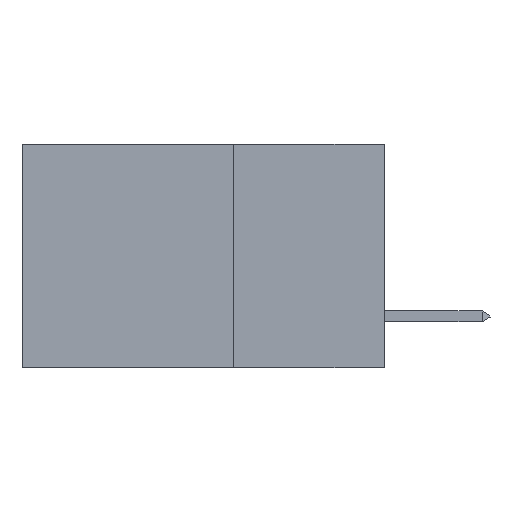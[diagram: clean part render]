
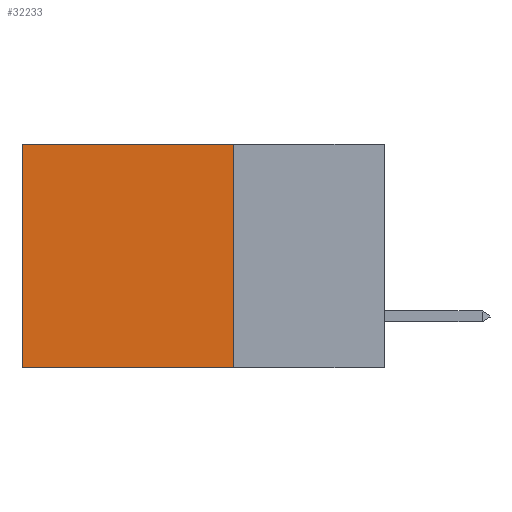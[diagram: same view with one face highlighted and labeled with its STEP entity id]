
A CAD part, left-side view. The second image highlights one B-rep face of the part: STEP entity #32233.
In plain terms, the highlighted planar face has unit normal (-1, 0, 0).
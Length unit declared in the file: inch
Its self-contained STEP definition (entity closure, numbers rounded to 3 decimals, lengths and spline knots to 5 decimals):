
#1003 = AXIS2_PLACEMENT_3D ( 'NONE', #18089, #18244, #40025 ) ;
#1364 = ORIENTED_EDGE ( 'NONE', *, *, #28501, .T. ) ;
#3052 = VECTOR ( 'NONE', #9744, 39.37008 ) ;
#4587 = VERTEX_POINT ( 'NONE', #31347 ) ;
#9744 = DIRECTION ( 'NONE',  ( 0., 1., 0. ) ) ;
#14249 = ORIENTED_EDGE ( 'NONE', *, *, #17210, .T. ) ;
#17210 = EDGE_CURVE ( 'NONE', #38135, #40889, #18634, .T. ) ;
#17909 = FACE_OUTER_BOUND ( 'NONE', #19977, .T. ) ;
#18089 = CARTESIAN_POINT ( 'NONE',  ( 0.2875, 0.25, 0. ) ) ;
#18244 = DIRECTION ( 'NONE',  ( 1., 0., 0. ) ) ;
#18634 = LINE ( 'NONE', #40462, #43501 ) ;
#19292 = VERTEX_POINT ( 'NONE', #30946 ) ;
#19977 = EDGE_LOOP ( 'NONE', ( #14249, #39201, #27418, #1364 ) ) ;
#21229 = CARTESIAN_POINT ( 'NONE',  ( 0.2875, 0.25, 0. ) ) ;
#24966 = DIRECTION ( 'NONE',  ( 0., 0., -1. ) ) ;
#27418 = ORIENTED_EDGE ( 'NONE', *, *, #46588, .F. ) ;
#28501 = EDGE_CURVE ( 'NONE', #19292, #38135, #42936, .T. ) ;
#30493 = CARTESIAN_POINT ( 'NONE',  ( 0.2875, 0.25, 0. ) ) ;
#30946 = CARTESIAN_POINT ( 'NONE',  ( 0.2875, 0.25, 0. ) ) ;
#31347 = CARTESIAN_POINT ( 'NONE',  ( 0.2875, 0.25, -0.37 ) ) ;
#32233 = ADVANCED_FACE ( 'NONE', ( #17909 ), #32477, .F. ) ;
#32477 = PLANE ( 'NONE',  #1003 ) ;
#32845 = CARTESIAN_POINT ( 'NONE',  ( 0.2875, 0.6, 0. ) ) ;
#33196 = VECTOR ( 'NONE', #24966, 39.37008 ) ;
#35670 = VECTOR ( 'NONE', #39908, 39.37008 ) ;
#36640 = LINE ( 'NONE', #21229, #33196 ) ;
#36789 = LINE ( 'NONE', #41172, #35670 ) ;
#37479 = EDGE_CURVE ( 'NONE', #4587, #40889, #36789, .T. ) ;
#38135 = VERTEX_POINT ( 'NONE', #32845 ) ;
#39201 = ORIENTED_EDGE ( 'NONE', *, *, #37479, .F. ) ;
#39563 = CARTESIAN_POINT ( 'NONE',  ( 0.2875, 0.6, -0.37 ) ) ;
#39908 = DIRECTION ( 'NONE',  ( 0., 1., 0. ) ) ;
#40025 = DIRECTION ( 'NONE',  ( 0., 0., -1. ) ) ;
#40462 = CARTESIAN_POINT ( 'NONE',  ( 0.2875, 0.6, 0. ) ) ;
#40889 = VERTEX_POINT ( 'NONE', #39563 ) ;
#41172 = CARTESIAN_POINT ( 'NONE',  ( 0.2875, 0.25, -0.37 ) ) ;
#42936 = LINE ( 'NONE', #30493, #3052 ) ;
#43501 = VECTOR ( 'NONE', #44483, 39.37008 ) ;
#44483 = DIRECTION ( 'NONE',  ( 0., 0., -1. ) ) ;
#46588 = EDGE_CURVE ( 'NONE', #19292, #4587, #36640, .T. ) ;
